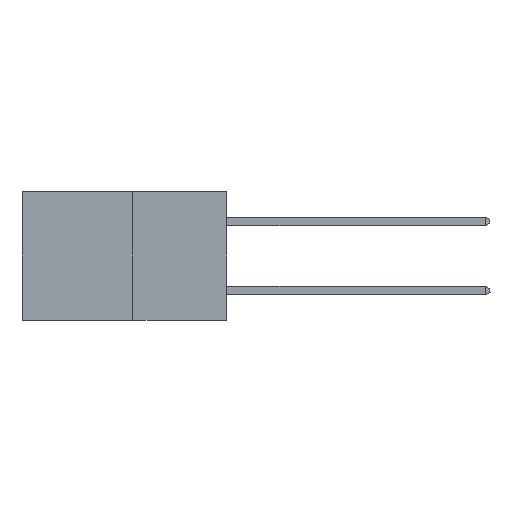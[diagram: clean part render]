
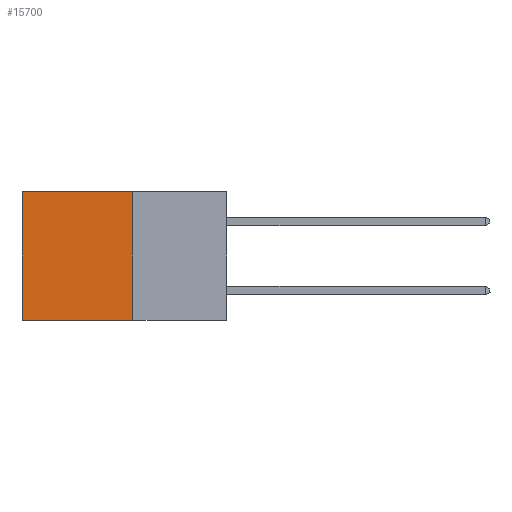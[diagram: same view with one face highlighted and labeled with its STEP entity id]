
A CAD part, left-side view. The second image highlights one B-rep face of the part: STEP entity #15700.
In plain terms, the highlighted planar face has unit normal (-1, 0, 0).
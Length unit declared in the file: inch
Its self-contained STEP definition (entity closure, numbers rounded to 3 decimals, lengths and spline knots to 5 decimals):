
#743 = AXIS2_PLACEMENT_3D ( 'NONE', #9803, #10515, #11397 ) ;
#1938 = DIRECTION ( 'NONE',  ( 0., 1., 0. ) ) ;
#3578 = LINE ( 'NONE', #5292, #11234 ) ;
#3601 = VERTEX_POINT ( 'NONE', #10780 ) ;
#3635 = ORIENTED_EDGE ( 'NONE', *, *, #10338, .F. ) ;
#4217 = VECTOR ( 'NONE', #13372, 39.37008 ) ;
#4237 = CARTESIAN_POINT ( 'NONE',  ( 0.277, 0.59, -0.37 ) ) ;
#5292 = CARTESIAN_POINT ( 'NONE',  ( 0.277, 0.27, 0. ) ) ;
#5675 = ORIENTED_EDGE ( 'NONE', *, *, #20239, .T. ) ;
#6076 = ORIENTED_EDGE ( 'NONE', *, *, #6085, .F. ) ;
#6085 = EDGE_CURVE ( 'NONE', #3601, #12690, #13943, .T. ) ;
#6964 = CARTESIAN_POINT ( 'NONE',  ( 0.277, 0.59, -0.37 ) ) ;
#7249 = VECTOR ( 'NONE', #17674, 39.37008 ) ;
#7786 = LINE ( 'NONE', #16118, #7249 ) ;
#8705 = EDGE_LOOP ( 'NONE', ( #15031, #3635, #6076, #5675 ) ) ;
#8812 = VERTEX_POINT ( 'NONE', #4237 ) ;
#9136 = EDGE_CURVE ( 'NONE', #16561, #8812, #12844, .T. ) ;
#9803 = CARTESIAN_POINT ( 'NONE',  ( 0.277, 0.27, -0.37 ) ) ;
#10338 = EDGE_CURVE ( 'NONE', #12690, #8812, #7786, .T. ) ;
#10515 = DIRECTION ( 'NONE',  ( 1., 0., 0. ) ) ;
#10780 = CARTESIAN_POINT ( 'NONE',  ( 0.277, 0.27, 0. ) ) ;
#11234 = VECTOR ( 'NONE', #1938, 39.37008 ) ;
#11397 = DIRECTION ( 'NONE',  ( 0., 0., -1. ) ) ;
#12690 = VERTEX_POINT ( 'NONE', #16281 ) ;
#12802 = CARTESIAN_POINT ( 'NONE',  ( 0.277, 0.27, -0.37 ) ) ;
#12844 = LINE ( 'NONE', #6964, #4217 ) ;
#12845 = DIRECTION ( 'NONE',  ( 0., 0., -1. ) ) ;
#12864 = PLANE ( 'NONE',  #743 ) ;
#13321 = CARTESIAN_POINT ( 'NONE',  ( 0.277, 0.59, 0. ) ) ;
#13372 = DIRECTION ( 'NONE',  ( 0., 0., -1. ) ) ;
#13943 = LINE ( 'NONE', #12802, #14447 ) ;
#14447 = VECTOR ( 'NONE', #12845, 39.37008 ) ;
#15031 = ORIENTED_EDGE ( 'NONE', *, *, #9136, .T. ) ;
#15700 = ADVANCED_FACE ( 'NONE', ( #17148 ), #12864, .F. ) ;
#16118 = CARTESIAN_POINT ( 'NONE',  ( 0.277, 0.27, -0.37 ) ) ;
#16281 = CARTESIAN_POINT ( 'NONE',  ( 0.277, 0.27, -0.37 ) ) ;
#16561 = VERTEX_POINT ( 'NONE', #13321 ) ;
#17148 = FACE_OUTER_BOUND ( 'NONE', #8705, .T. ) ;
#17674 = DIRECTION ( 'NONE',  ( 0., 1., 0. ) ) ;
#20239 = EDGE_CURVE ( 'NONE', #3601, #16561, #3578, .T. ) ;
